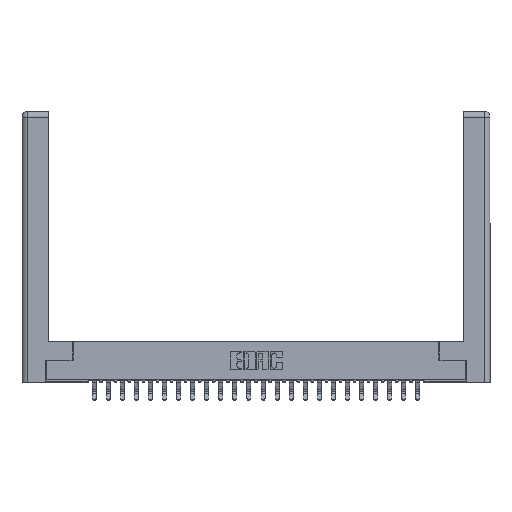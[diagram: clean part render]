
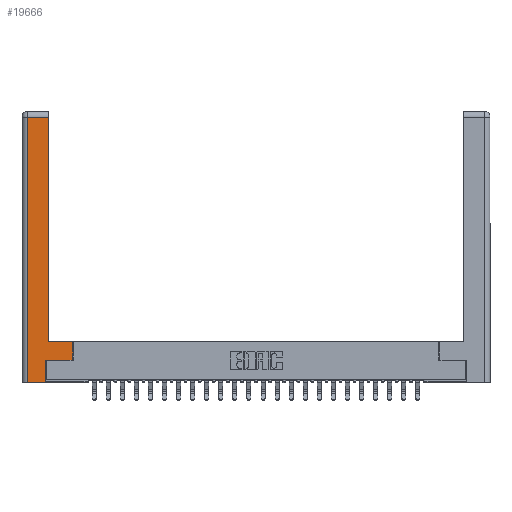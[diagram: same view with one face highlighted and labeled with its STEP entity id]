
A CAD part, top view. The second image highlights one B-rep face of the part: STEP entity #19666.
In plain terms, the highlighted planar face has unit normal (0, 0, 1).
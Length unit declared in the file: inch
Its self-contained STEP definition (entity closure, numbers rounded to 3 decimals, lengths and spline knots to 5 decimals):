
#179 = ORIENTED_EDGE ( 'NONE', *, *, #12773, .T. ) ;
#487 = CARTESIAN_POINT ( 'NONE',  ( 0.265, 0.245, 0. ) ) ;
#793 = VECTOR ( 'NONE', #13403, 39.37008 ) ;
#1070 = VECTOR ( 'NONE', #5613, 39.37008 ) ;
#1251 = CARTESIAN_POINT ( 'NONE',  ( 0.0615, 0., 0. ) ) ;
#2285 = VECTOR ( 'NONE', #3959, 39.37008 ) ;
#3077 = CARTESIAN_POINT ( 'NONE',  ( 0.265, 0.245, 0. ) ) ;
#3251 = EDGE_CURVE ( 'NONE', #9765, #4511, #25784, .T. ) ;
#3565 = DIRECTION ( 'NONE',  ( -1., 0., 0. ) ) ;
#3709 = DIRECTION ( 'NONE',  ( 0., 1., 0. ) ) ;
#3855 = VERTEX_POINT ( 'NONE', #25798 ) ;
#3870 = CARTESIAN_POINT ( 'NONE',  ( 0.295, 0.45, 0. ) ) ;
#3910 = LINE ( 'NONE', #3870, #26717 ) ;
#3959 = DIRECTION ( 'NONE',  ( 1., 0., 0. ) ) ;
#4281 = VERTEX_POINT ( 'NONE', #25814 ) ;
#4511 = VERTEX_POINT ( 'NONE', #1251 ) ;
#5613 = DIRECTION ( 'NONE',  ( 0., 1., 0. ) ) ;
#6042 = CARTESIAN_POINT ( 'NONE',  ( 0.295, 3., 0. ) ) ;
#6309 = CARTESIAN_POINT ( 'NONE',  ( 0.565, 0.245, 0. ) ) ;
#6971 = EDGE_CURVE ( 'NONE', #3855, #15337, #17702, .T. ) ;
#7150 = VERTEX_POINT ( 'NONE', #487 ) ;
#7248 = ORIENTED_EDGE ( 'NONE', *, *, #6971, .T. ) ;
#7348 = DIRECTION ( 'NONE',  ( 0., 0., -1. ) ) ;
#8786 = LINE ( 'NONE', #17054, #24450 ) ;
#9593 = DIRECTION ( 'NONE',  ( -1., 0., 0. ) ) ;
#9765 = VERTEX_POINT ( 'NONE', #14459 ) ;
#9883 = VERTEX_POINT ( 'NONE', #27365 ) ;
#10491 = ORIENTED_EDGE ( 'NONE', *, *, #13122, .T. ) ;
#11019 = EDGE_CURVE ( 'NONE', #15337, #9765, #8786, .T. ) ;
#11932 = VECTOR ( 'NONE', #24879, 39.37008 ) ;
#12773 = EDGE_CURVE ( 'NONE', #26244, #9883, #22494, .T. ) ;
#13122 = EDGE_CURVE ( 'NONE', #9883, #3855, #3910, .T. ) ;
#13403 = DIRECTION ( 'NONE',  ( 0., 1., 0. ) ) ;
#13842 = VECTOR ( 'NONE', #25073, 39.37008 ) ;
#14038 = ORIENTED_EDGE ( 'NONE', *, *, #20560, .T. ) ;
#14459 = CARTESIAN_POINT ( 'NONE',  ( 0.0615, 2.94, 0. ) ) ;
#14523 = PLANE ( 'NONE',  #25929 ) ;
#15337 = VERTEX_POINT ( 'NONE', #25190 ) ;
#16062 = ORIENTED_EDGE ( 'NONE', *, *, #11019, .T. ) ;
#16782 = CARTESIAN_POINT ( 'NONE',  ( 0., 0., 0. ) ) ;
#17054 = CARTESIAN_POINT ( 'NONE',  ( 0.0615, 2.94, 0. ) ) ;
#17702 = LINE ( 'NONE', #6042, #30099 ) ;
#18443 = CARTESIAN_POINT ( 'NONE',  ( 0.265, 0., 0. ) ) ;
#19065 = DIRECTION ( 'NONE',  ( -1., 0., 0. ) ) ;
#19666 = ADVANCED_FACE ( 'NONE', ( #22870 ), #14523, .F. ) ;
#20128 = LINE ( 'NONE', #21883, #11932 ) ;
#20560 = EDGE_CURVE ( 'NONE', #4511, #4281, #28057, .T. ) ;
#20586 = CARTESIAN_POINT ( 'NONE',  ( 0.0615, 0., 0. ) ) ;
#21883 = CARTESIAN_POINT ( 'NONE',  ( 0.565, 0.245, 0. ) ) ;
#22206 = EDGE_CURVE ( 'NONE', #4281, #7150, #24225, .T. ) ;
#22494 = LINE ( 'NONE', #25078, #793 ) ;
#22620 = ORIENTED_EDGE ( 'NONE', *, *, #22772, .T. ) ;
#22772 = EDGE_CURVE ( 'NONE', #7150, #26244, #20128, .T. ) ;
#22870 = FACE_OUTER_BOUND ( 'NONE', #24870, .T. ) ;
#24225 = LINE ( 'NONE', #3077, #1070 ) ;
#24450 = VECTOR ( 'NONE', #9593, 39.37008 ) ;
#24476 = ORIENTED_EDGE ( 'NONE', *, *, #22206, .T. ) ;
#24870 = EDGE_LOOP ( 'NONE', ( #7248, #16062, #29221, #14038, #24476, #22620, #179, #10491 ) ) ;
#24879 = DIRECTION ( 'NONE',  ( 1., 0., 0. ) ) ;
#25073 = DIRECTION ( 'NONE',  ( 0., -1., 0. ) ) ;
#25078 = CARTESIAN_POINT ( 'NONE',  ( 0.565, 0.45, 0. ) ) ;
#25190 = CARTESIAN_POINT ( 'NONE',  ( 0.295, 2.94, 0. ) ) ;
#25784 = LINE ( 'NONE', #20586, #13842 ) ;
#25798 = CARTESIAN_POINT ( 'NONE',  ( 0.295, 0.45, 0. ) ) ;
#25814 = CARTESIAN_POINT ( 'NONE',  ( 0.265, 0., 0. ) ) ;
#25929 = AXIS2_PLACEMENT_3D ( 'NONE', #16782, #7348, #19065 ) ;
#26244 = VERTEX_POINT ( 'NONE', #6309 ) ;
#26717 = VECTOR ( 'NONE', #3565, 39.37008 ) ;
#27365 = CARTESIAN_POINT ( 'NONE',  ( 0.565, 0.45, 0. ) ) ;
#28057 = LINE ( 'NONE', #18443, #2285 ) ;
#29221 = ORIENTED_EDGE ( 'NONE', *, *, #3251, .T. ) ;
#30099 = VECTOR ( 'NONE', #3709, 39.37008 ) ;
